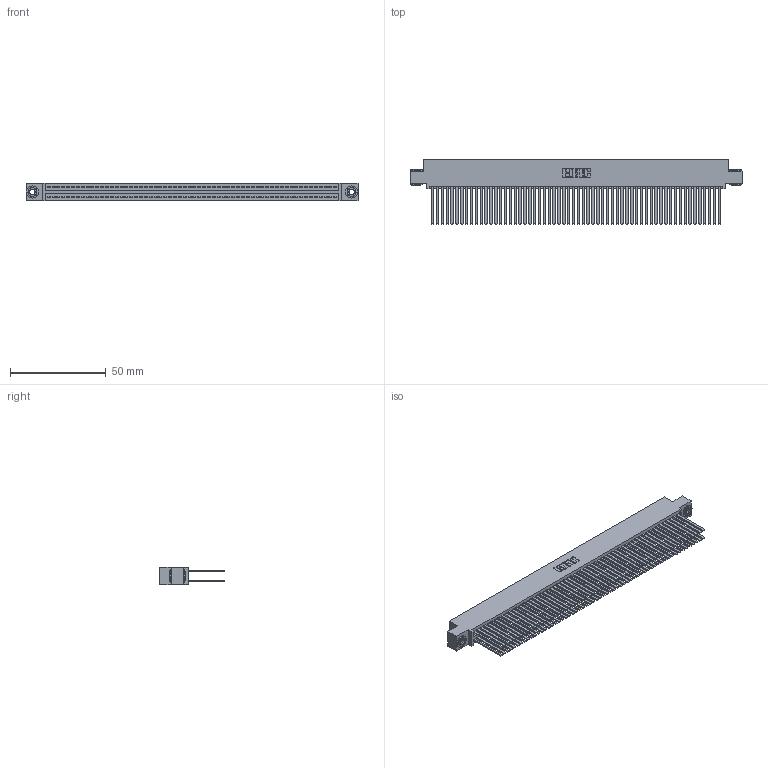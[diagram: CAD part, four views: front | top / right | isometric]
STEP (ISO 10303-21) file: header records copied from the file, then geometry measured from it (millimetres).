
FILE_DESCRIPTION (( 'STEP AP203' ), '1' );
FILE_NAME ('845-120-544-503.STEP', '2018-11-21T04:49:42', ( '' ), ( '' ), 'SwSTEP 2.0', 'SolidWorks 2016', '' );
FILE_SCHEMA (( 'CONFIG_CONTROL_DESIGN' ));
Length unit declared in the file: inch
Products named in the file (4): 845 Part_0.110 Offset - 0.156 Dia-TH; 345-292-001_345-293-144; 345-250-002_345-250-002-102; 845-120-544-503
Assembly tree (123 placements, depth 2):
  845-120-544-503
    845 Part_0.110 Offset - 0.156 Dia-TH
    345-292-001_345-293-144  x120
    345-250-002_345-250-002-102  x2
Bounding box: 173.61 x 33.96 x 9.4 mm (x, y, z)
Volume: 18659.8 mm3; surface area: 33159.1 mm2
Topology: 123 solids, 123 shells, 5448 faces, 16149 edges, 10602 vertices
Faces by surface type: plane 3574, cylinder 1866, cone 8
Entity records: 45252 total; most frequent: CARTESIAN_POINT 7543, ORIENTED_EDGE 7470, DIRECTION 6657, EDGE_CURVE 3735, LINE 3343, VECTOR 3343, VERTEX_POINT 2486, AXIS2_PLACEMENT_3D 1657
